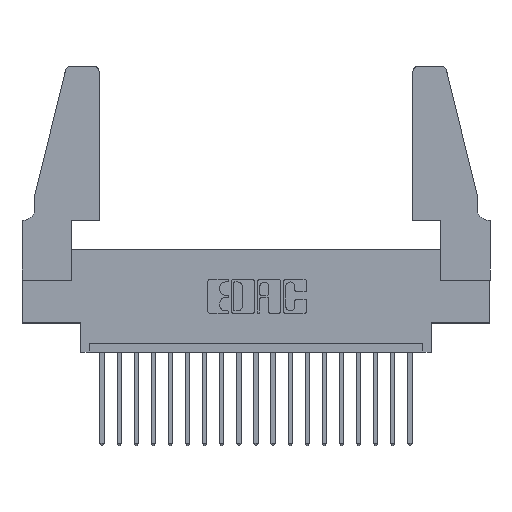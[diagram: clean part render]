
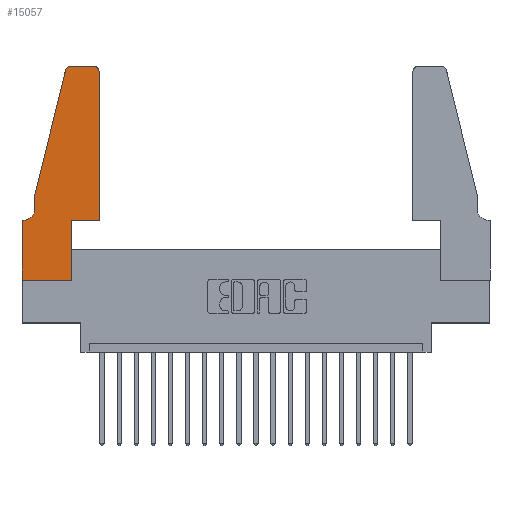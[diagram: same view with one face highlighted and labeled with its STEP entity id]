
A CAD part, top view. The second image highlights one B-rep face of the part: STEP entity #15057.
In plain terms, the highlighted planar face has unit normal (0, 0, 1).
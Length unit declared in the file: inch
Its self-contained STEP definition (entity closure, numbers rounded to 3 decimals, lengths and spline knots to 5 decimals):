
#341 = LINE ( 'NONE', #16063, #3446 ) ;
#562 = DIRECTION ( 'NONE',  ( -0.239, -0.971, 0. ) ) ;
#760 = EDGE_CURVE ( 'NONE', #16351, #15506, #17994, .T. ) ;
#1003 = EDGE_CURVE ( 'NONE', #5082, #18318, #2558, .T. ) ;
#1077 = VERTEX_POINT ( 'NONE', #11331 ) ;
#1209 = CARTESIAN_POINT ( 'NONE',  ( 0.25487, 1.22718, 0.37 ) ) ;
#1634 = CARTESIAN_POINT ( 'NONE',  ( 0., 0.35, 0.37 ) ) ;
#1848 = EDGE_CURVE ( 'NONE', #5006, #5082, #18199, .T. ) ;
#1957 = AXIS2_PLACEMENT_3D ( 'NONE', #17885, #4412, #11856 ) ;
#1985 = CARTESIAN_POINT ( 'NONE',  ( 0.2865, 0.35, 0.37 ) ) ;
#2078 = ORIENTED_EDGE ( 'NONE', *, *, #760, .T. ) ;
#2253 = PLANE ( 'NONE',  #9249 ) ;
#2336 = CARTESIAN_POINT ( 'NONE',  ( 0.4205, 1.25, 0.37 ) ) ;
#2558 = LINE ( 'NONE', #6355, #13717 ) ;
#2637 = VERTEX_POINT ( 'NONE', #17704 ) ;
#3229 = VECTOR ( 'NONE', #8383, 39.37008 ) ;
#3244 = VECTOR ( 'NONE', #12032, 39.37008 ) ;
#3314 = EDGE_CURVE ( 'NONE', #16039, #2637, #13625, .T. ) ;
#3446 = VECTOR ( 'NONE', #3978, 39.37008 ) ;
#3563 = ORIENTED_EDGE ( 'NONE', *, *, #11083, .T. ) ;
#3660 = CARTESIAN_POINT ( 'NONE',  ( 0., 0.35, 0.37 ) ) ;
#3978 = DIRECTION ( 'NONE',  ( 0., -1., 0. ) ) ;
#3986 = CARTESIAN_POINT ( 'NONE',  ( 0.0755, 0.5, 0.37 ) ) ;
#4412 = DIRECTION ( 'NONE',  ( 0., 0., 1. ) ) ;
#4466 = VECTOR ( 'NONE', #13232, 39.37008 ) ;
#4535 = ORIENTED_EDGE ( 'NONE', *, *, #1848, .T. ) ;
#4660 = VERTEX_POINT ( 'NONE', #11790 ) ;
#4856 = LINE ( 'NONE', #19695, #18150 ) ;
#4958 = DIRECTION ( 'NONE',  ( -1., 0., 0. ) ) ;
#5006 = VERTEX_POINT ( 'NONE', #1985 ) ;
#5082 = VERTEX_POINT ( 'NONE', #8368 ) ;
#5107 = DIRECTION ( 'NONE',  ( 0., 0., 1. ) ) ;
#5443 = CARTESIAN_POINT ( 'NONE',  ( 0.0055, 0.35, 0.37 ) ) ;
#5740 = CARTESIAN_POINT ( 'NONE',  ( 0.4505, 1.22, 0.37 ) ) ;
#6047 = CIRCLE ( 'NONE', #12764, 0.03 ) ;
#6355 = CARTESIAN_POINT ( 'NONE',  ( 0.4505, 0.35, 0.37 ) ) ;
#6933 = VERTEX_POINT ( 'NONE', #9877 ) ;
#7154 = ORIENTED_EDGE ( 'NONE', *, *, #10298, .T. ) ;
#7246 = EDGE_CURVE ( 'NONE', #4660, #1077, #9225, .T. ) ;
#8158 = ORIENTED_EDGE ( 'NONE', *, *, #10875, .T. ) ;
#8317 = ORIENTED_EDGE ( 'NONE', *, *, #7246, .T. ) ;
#8368 = CARTESIAN_POINT ( 'NONE',  ( 0.4505, 0.35, 0.37 ) ) ;
#8383 = DIRECTION ( 'NONE',  ( 0., -1., 0. ) ) ;
#9225 = LINE ( 'NONE', #16234, #4466 ) ;
#9244 = EDGE_CURVE ( 'NONE', #18318, #18813, #6047, .T. ) ;
#9249 = AXIS2_PLACEMENT_3D ( 'NONE', #3660, #5107, #17190 ) ;
#9394 = DIRECTION ( 'NONE',  ( -1., 0., 0. ) ) ;
#9406 = CARTESIAN_POINT ( 'NONE',  ( 0.4205, 1.22, 0.37 ) ) ;
#9607 = VECTOR ( 'NONE', #562, 39.37008 ) ;
#9877 = CARTESIAN_POINT ( 'NONE',  ( 0.284, 1.25, 0.37 ) ) ;
#10298 = EDGE_CURVE ( 'NONE', #15506, #4660, #341, .T. ) ;
#10522 = CIRCLE ( 'NONE', #1957, 0.03 ) ;
#10684 = CIRCLE ( 'NONE', #19255, 0.07 ) ;
#10875 = EDGE_CURVE ( 'NONE', #6933, #16039, #10522, .T. ) ;
#10928 = ORIENTED_EDGE ( 'NONE', *, *, #16041, .T. ) ;
#11083 = EDGE_CURVE ( 'NONE', #18813, #6933, #15291, .T. ) ;
#11253 = VECTOR ( 'NONE', #4958, 39.37008 ) ;
#11268 = DIRECTION ( 'NONE',  ( 0., 0., -1. ) ) ;
#11331 = CARTESIAN_POINT ( 'NONE',  ( 0.2865, 0., 0.37 ) ) ;
#11772 = LINE ( 'NONE', #3986, #3229 ) ;
#11790 = CARTESIAN_POINT ( 'NONE',  ( 0., 0., 0.37 ) ) ;
#11856 = DIRECTION ( 'NONE',  ( 1., 0., 0. ) ) ;
#12032 = DIRECTION ( 'NONE',  ( 1., 0., 0. ) ) ;
#12466 = DIRECTION ( 'NONE',  ( 0., 0., 1. ) ) ;
#12639 = EDGE_CURVE ( 'NONE', #18090, #16351, #10684, .T. ) ;
#12764 = AXIS2_PLACEMENT_3D ( 'NONE', #9406, #12466, #13971 ) ;
#12976 = ORIENTED_EDGE ( 'NONE', *, *, #1003, .T. ) ;
#13232 = DIRECTION ( 'NONE',  ( 1., 0., 0. ) ) ;
#13555 = DIRECTION ( 'NONE',  ( 0., 1., 0. ) ) ;
#13625 = LINE ( 'NONE', #17091, #9607 ) ;
#13717 = VECTOR ( 'NONE', #15548, 39.37008 ) ;
#13756 = ORIENTED_EDGE ( 'NONE', *, *, #17525, .T. ) ;
#13971 = DIRECTION ( 'NONE',  ( 1., 0., 0. ) ) ;
#14116 = CARTESIAN_POINT ( 'NONE',  ( 0.0055, 0.42, 0.37 ) ) ;
#14309 = CARTESIAN_POINT ( 'NONE',  ( 0.0755, 0.42, 0.37 ) ) ;
#14962 = CARTESIAN_POINT ( 'NONE',  ( 0.0755, 0.35, 0.37 ) ) ;
#15006 = CARTESIAN_POINT ( 'NONE',  ( 0.4505, 0.35, 0.37 ) ) ;
#15057 = ADVANCED_FACE ( 'NONE', ( #15619 ), #2253, .T. ) ;
#15213 = ORIENTED_EDGE ( 'NONE', *, *, #12639, .T. ) ;
#15291 = LINE ( 'NONE', #17052, #11253 ) ;
#15506 = VERTEX_POINT ( 'NONE', #1634 ) ;
#15548 = DIRECTION ( 'NONE',  ( 0., 1., 0. ) ) ;
#15619 = FACE_OUTER_BOUND ( 'NONE', #18880, .T. ) ;
#15743 = ORIENTED_EDGE ( 'NONE', *, *, #3314, .T. ) ;
#15854 = DIRECTION ( 'NONE',  ( -1., 0., 0. ) ) ;
#16039 = VERTEX_POINT ( 'NONE', #1209 ) ;
#16041 = EDGE_CURVE ( 'NONE', #1077, #5006, #4856, .T. ) ;
#16063 = CARTESIAN_POINT ( 'NONE',  ( 0., 0., 0.37 ) ) ;
#16234 = CARTESIAN_POINT ( 'NONE',  ( 0., 0., 0.37 ) ) ;
#16351 = VERTEX_POINT ( 'NONE', #5443 ) ;
#17052 = CARTESIAN_POINT ( 'NONE',  ( 0.2605, 1.25, 0.37 ) ) ;
#17091 = CARTESIAN_POINT ( 'NONE',  ( 0.0755, 0.5, 0.37 ) ) ;
#17190 = DIRECTION ( 'NONE',  ( 1., 0., 0. ) ) ;
#17525 = EDGE_CURVE ( 'NONE', #2637, #18090, #11772, .T. ) ;
#17704 = CARTESIAN_POINT ( 'NONE',  ( 0.0755, 0.5, 0.37 ) ) ;
#17885 = CARTESIAN_POINT ( 'NONE',  ( 0.284, 1.22, 0.37 ) ) ;
#17994 = LINE ( 'NONE', #14962, #18236 ) ;
#18090 = VERTEX_POINT ( 'NONE', #14309 ) ;
#18150 = VECTOR ( 'NONE', #13555, 39.37008 ) ;
#18199 = LINE ( 'NONE', #15006, #3244 ) ;
#18236 = VECTOR ( 'NONE', #9394, 39.37008 ) ;
#18318 = VERTEX_POINT ( 'NONE', #5740 ) ;
#18813 = VERTEX_POINT ( 'NONE', #2336 ) ;
#18880 = EDGE_LOOP ( 'NONE', ( #3563, #8158, #15743, #13756, #15213, #2078, #7154, #8317, #10928, #4535, #12976, #19415 ) ) ;
#19255 = AXIS2_PLACEMENT_3D ( 'NONE', #14116, #11268, #15854 ) ;
#19415 = ORIENTED_EDGE ( 'NONE', *, *, #9244, .T. ) ;
#19695 = CARTESIAN_POINT ( 'NONE',  ( 0.2865, 0.35, 0.37 ) ) ;
